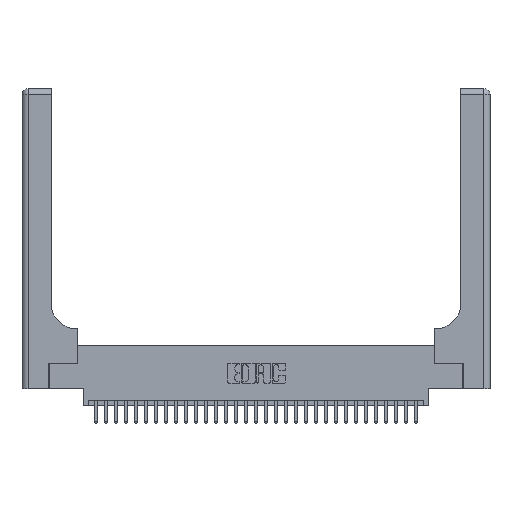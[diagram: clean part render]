
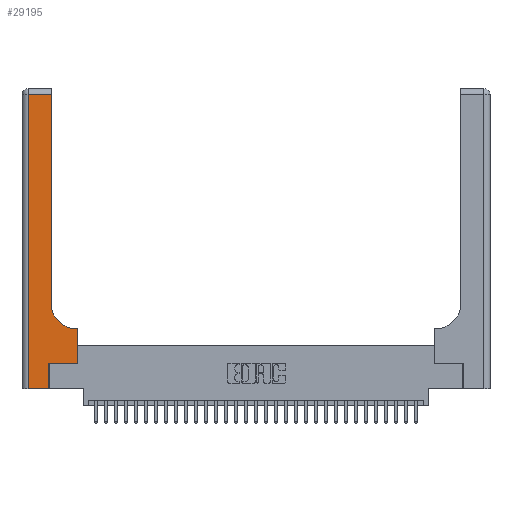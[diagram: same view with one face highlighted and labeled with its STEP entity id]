
A CAD part, top view. The second image highlights one B-rep face of the part: STEP entity #29195.
In plain terms, the highlighted planar face has unit normal (0, 0, 1).
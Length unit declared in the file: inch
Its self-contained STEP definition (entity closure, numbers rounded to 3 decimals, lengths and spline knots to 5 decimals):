
#133 = VERTEX_POINT ( 'NONE', #30139 ) ;
#296 = VECTOR ( 'NONE', #26786, 39.37008 ) ;
#636 = DIRECTION ( 'NONE',  ( 1., 0., 0. ) ) ;
#2395 = LINE ( 'NONE', #9279, #29921 ) ;
#2999 = ORIENTED_EDGE ( 'NONE', *, *, #24252, .T. ) ;
#3317 = DIRECTION ( 'NONE',  ( 0., 0., -1. ) ) ;
#4270 = EDGE_CURVE ( 'NONE', #5211, #133, #2395, .T. ) ;
#4283 = LINE ( 'NONE', #5778, #21091 ) ;
#4891 = CARTESIAN_POINT ( 'NONE',  ( 0., 2.94, 0.37 ) ) ;
#5036 = AXIS2_PLACEMENT_3D ( 'NONE', #30441, #3317, #636 ) ;
#5211 = VERTEX_POINT ( 'NONE', #32441 ) ;
#5378 = EDGE_CURVE ( 'NONE', #28898, #22848, #25496, .T. ) ;
#5553 = DIRECTION ( 'NONE',  ( 0., -1., 0. ) ) ;
#5778 = CARTESIAN_POINT ( 'NONE',  ( 0.269, 0., 0.37 ) ) ;
#6087 = CARTESIAN_POINT ( 'NONE',  ( 0., 3., 0.37 ) ) ;
#6431 = CARTESIAN_POINT ( 'NONE',  ( 0.2915, 0.6, 0.37 ) ) ;
#6724 = FACE_OUTER_BOUND ( 'NONE', #13673, .T. ) ;
#7176 = EDGE_CURVE ( 'NONE', #15229, #28898, #14781, .T. ) ;
#7672 = AXIS2_PLACEMENT_3D ( 'NONE', #6087, #18211, #23342 ) ;
#7994 = CARTESIAN_POINT ( 'NONE',  ( 0.5585, 0.6, 0.37 ) ) ;
#8188 = VECTOR ( 'NONE', #17556, 39.37008 ) ;
#9197 = CARTESIAN_POINT ( 'NONE',  ( 0.06, 2.94, 0.37 ) ) ;
#9279 = CARTESIAN_POINT ( 'NONE',  ( 0.2915, 3., 0.37 ) ) ;
#10241 = DIRECTION ( 'NONE',  ( 0., 1., 0. ) ) ;
#10468 = ORIENTED_EDGE ( 'NONE', *, *, #26982, .T. ) ;
#10676 = CARTESIAN_POINT ( 'NONE',  ( 0.269, 0., 0.37 ) ) ;
#11182 = VECTOR ( 'NONE', #5553, 39.37008 ) ;
#11318 = CARTESIAN_POINT ( 'NONE',  ( 0.5415, 0.6, 0.37 ) ) ;
#11373 = EDGE_CURVE ( 'NONE', #31001, #28131, #28622, .T. ) ;
#11668 = CARTESIAN_POINT ( 'NONE',  ( 0.06, 3., 0.37 ) ) ;
#11826 = CARTESIAN_POINT ( 'NONE',  ( 0., 0., 0.37 ) ) ;
#12187 = CARTESIAN_POINT ( 'NONE',  ( 0.269, 0.25, 0.37 ) ) ;
#13473 = ORIENTED_EDGE ( 'NONE', *, *, #22111, .T. ) ;
#13673 = EDGE_LOOP ( 'NONE', ( #25599, #31293, #30184, #21724, #13706, #10468, #2999, #16072, #13473 ) ) ;
#13706 = ORIENTED_EDGE ( 'NONE', *, *, #15136, .T. ) ;
#14781 = LINE ( 'NONE', #11668, #11182 ) ;
#15136 = EDGE_CURVE ( 'NONE', #22848, #26925, #4283, .T. ) ;
#15229 = VERTEX_POINT ( 'NONE', #9197 ) ;
#16072 = ORIENTED_EDGE ( 'NONE', *, *, #11373, .T. ) ;
#16704 = DIRECTION ( 'NONE',  ( -1., 0., 0. ) ) ;
#17556 = DIRECTION ( 'NONE',  ( -1., 0., 0. ) ) ;
#18211 = DIRECTION ( 'NONE',  ( 0., 0., -1. ) ) ;
#18417 = VECTOR ( 'NONE', #16704, 39.37008 ) ;
#19082 = VECTOR ( 'NONE', #27241, 39.37008 ) ;
#19863 = LINE ( 'NONE', #29432, #19082 ) ;
#21091 = VECTOR ( 'NONE', #28531, 39.37008 ) ;
#21116 = PLANE ( 'NONE',  #7672 ) ;
#21724 = ORIENTED_EDGE ( 'NONE', *, *, #5378, .T. ) ;
#21906 = CARTESIAN_POINT ( 'NONE',  ( 0.5585, 0.25, 0.37 ) ) ;
#21950 = LINE ( 'NONE', #21906, #296 ) ;
#22111 = EDGE_CURVE ( 'NONE', #28131, #5211, #26451, .T. ) ;
#22848 = VERTEX_POINT ( 'NONE', #10676 ) ;
#23342 = DIRECTION ( 'NONE',  ( -1., 0., 0. ) ) ;
#24252 = EDGE_CURVE ( 'NONE', #24426, #31001, #21950, .T. ) ;
#24393 = EDGE_CURVE ( 'NONE', #133, #15229, #28605, .T. ) ;
#24426 = VERTEX_POINT ( 'NONE', #29949 ) ;
#25496 = LINE ( 'NONE', #11826, #30579 ) ;
#25599 = ORIENTED_EDGE ( 'NONE', *, *, #4270, .T. ) ;
#26451 = CIRCLE ( 'NONE', #5036, 0.25 ) ;
#26774 = DIRECTION ( 'NONE',  ( 1., 0., 0. ) ) ;
#26786 = DIRECTION ( 'NONE',  ( 0., 1., 0. ) ) ;
#26925 = VERTEX_POINT ( 'NONE', #12187 ) ;
#26982 = EDGE_CURVE ( 'NONE', #26925, #24426, #19863, .T. ) ;
#27241 = DIRECTION ( 'NONE',  ( 1., 0., 0. ) ) ;
#28131 = VERTEX_POINT ( 'NONE', #11318 ) ;
#28531 = DIRECTION ( 'NONE',  ( 0., 1., 0. ) ) ;
#28605 = LINE ( 'NONE', #4891, #8188 ) ;
#28622 = LINE ( 'NONE', #6431, #18417 ) ;
#28898 = VERTEX_POINT ( 'NONE', #29776 ) ;
#29195 = ADVANCED_FACE ( 'NONE', ( #6724 ), #21116, .F. ) ;
#29432 = CARTESIAN_POINT ( 'NONE',  ( 0.269, 0.25, 0.37 ) ) ;
#29776 = CARTESIAN_POINT ( 'NONE',  ( 0.06, 0., 0.37 ) ) ;
#29921 = VECTOR ( 'NONE', #10241, 39.37008 ) ;
#29949 = CARTESIAN_POINT ( 'NONE',  ( 0.5585, 0.25, 0.37 ) ) ;
#30139 = CARTESIAN_POINT ( 'NONE',  ( 0.2915, 2.94, 0.37 ) ) ;
#30184 = ORIENTED_EDGE ( 'NONE', *, *, #7176, .T. ) ;
#30441 = CARTESIAN_POINT ( 'NONE',  ( 0.5415, 0.85, 0.37 ) ) ;
#30579 = VECTOR ( 'NONE', #26774, 39.37008 ) ;
#31001 = VERTEX_POINT ( 'NONE', #7994 ) ;
#31293 = ORIENTED_EDGE ( 'NONE', *, *, #24393, .T. ) ;
#32441 = CARTESIAN_POINT ( 'NONE',  ( 0.2915, 0.85, 0.37 ) ) ;
